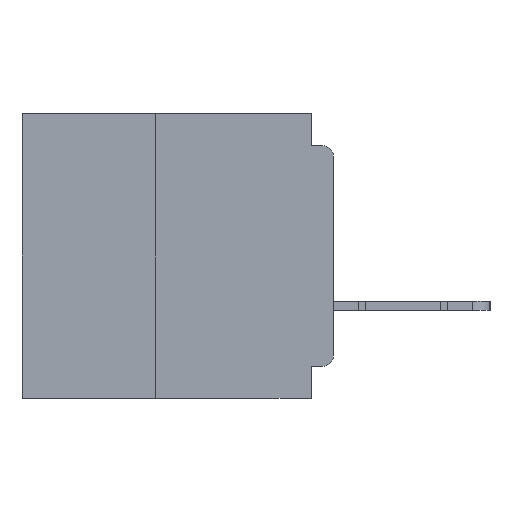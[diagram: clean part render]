
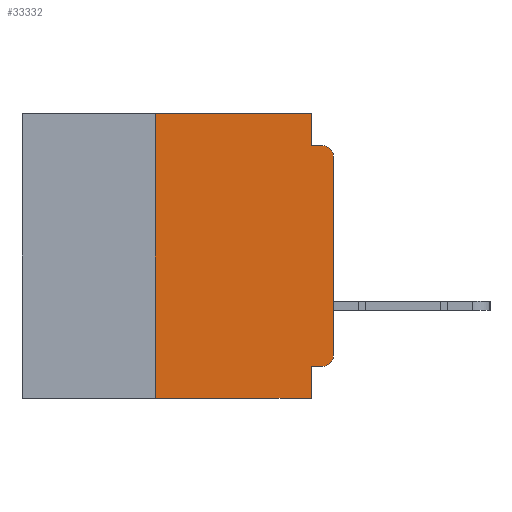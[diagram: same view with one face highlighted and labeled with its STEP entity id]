
A CAD part, left-side view. The second image highlights one B-rep face of the part: STEP entity #33332.
In plain terms, the highlighted planar face has unit normal (-1, 0, 0).
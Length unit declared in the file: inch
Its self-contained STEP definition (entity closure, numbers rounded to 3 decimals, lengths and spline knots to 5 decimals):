
#23 = VECTOR ( 'NONE', #9701, 39.37008 ) ;
#834 = EDGE_CURVE ( 'NONE', #57374, #1180, #47469, .T. ) ;
#1180 = VERTEX_POINT ( 'NONE', #57865 ) ;
#1313 = EDGE_CURVE ( 'NONE', #57374, #57992, #45757, .T. ) ;
#1717 = LINE ( 'NONE', #67734, #23 ) ;
#3343 = VECTOR ( 'NONE', #42000, 39.37008 ) ;
#3476 = DIRECTION ( 'NONE',  ( 0., 0., 1. ) ) ;
#3746 = DIRECTION ( 'NONE',  ( 0., 0., -1. ) ) ;
#3968 = DIRECTION ( 'NONE',  ( -1., 0., 0. ) ) ;
#3980 = CARTESIAN_POINT ( 'NONE',  ( 0., 0.015, -0.34 ) ) ;
#4348 = CARTESIAN_POINT ( 'NONE',  ( 0., 0.015, -0.045 ) ) ;
#5704 = CARTESIAN_POINT ( 'NONE',  ( 0., 0.031, -0.4 ) ) ;
#5742 = VERTEX_POINT ( 'NONE', #41278 ) ;
#6002 = ORIENTED_EDGE ( 'NONE', *, *, #11549, .T. ) ;
#6520 = EDGE_CURVE ( 'NONE', #5742, #25308, #28295, .T. ) ;
#7886 = VERTEX_POINT ( 'NONE', #61480 ) ;
#9701 = DIRECTION ( 'NONE',  ( 0., -1., 0. ) ) ;
#11549 = EDGE_CURVE ( 'NONE', #58336, #25308, #24708, .T. ) ;
#12817 = LINE ( 'NONE', #5704, #64125 ) ;
#13571 = EDGE_CURVE ( 'NONE', #1180, #58336, #45161, .T. ) ;
#14651 = VERTEX_POINT ( 'NONE', #18048 ) ;
#15087 = VECTOR ( 'NONE', #3476, 39.37008 ) ;
#15873 = VECTOR ( 'NONE', #26527, 39.37008 ) ;
#16516 = EDGE_CURVE ( 'NONE', #57992, #7886, #12817, .T. ) ;
#16991 = VECTOR ( 'NONE', #24159, 39.37008 ) ;
#17521 = CARTESIAN_POINT ( 'NONE',  ( 0., 0.031, 0. ) ) ;
#18048 = CARTESIAN_POINT ( 'NONE',  ( 0., 0.25, 0. ) ) ;
#21211 = CARTESIAN_POINT ( 'NONE',  ( 0., 0., -0.045 ) ) ;
#21913 = DIRECTION ( 'NONE',  ( 1., 0., 0. ) ) ;
#22072 = EDGE_CURVE ( 'NONE', #51188, #7886, #1717, .T. ) ;
#24159 = DIRECTION ( 'NONE',  ( 0., 0., 1. ) ) ;
#24708 = CIRCLE ( 'NONE', #51439, 0.015 ) ;
#25308 = VERTEX_POINT ( 'NONE', #4348 ) ;
#25977 = CARTESIAN_POINT ( 'NONE',  ( 0., 0.015, -0.355 ) ) ;
#26128 = CARTESIAN_POINT ( 'NONE',  ( 0., 0.031, -0.355 ) ) ;
#26527 = DIRECTION ( 'NONE',  ( 0., -1., 0. ) ) ;
#26719 = ORIENTED_EDGE ( 'NONE', *, *, #1313, .F. ) ;
#27508 = DIRECTION ( 'NONE',  ( 0., -1., 0. ) ) ;
#27667 = ORIENTED_EDGE ( 'NONE', *, *, #13571, .T. ) ;
#28295 = LINE ( 'NONE', #21211, #15873 ) ;
#30493 = AXIS2_PLACEMENT_3D ( 'NONE', #43035, #21913, #58931 ) ;
#31393 = CARTESIAN_POINT ( 'NONE',  ( 0., 0.015, -0.06 ) ) ;
#32190 = CARTESIAN_POINT ( 'NONE',  ( 0., 0.25, -0.4 ) ) ;
#33332 = ADVANCED_FACE ( 'NONE', ( #68121 ), #37674, .F. ) ;
#34059 = ORIENTED_EDGE ( 'NONE', *, *, #54883, .F. ) ;
#35324 = CARTESIAN_POINT ( 'NONE',  ( 0., 0.25, -0.4 ) ) ;
#36691 = DIRECTION ( 'NONE',  ( 0., 0., -1. ) ) ;
#37674 = PLANE ( 'NONE',  #30493 ) ;
#37801 = CARTESIAN_POINT ( 'NONE',  ( 0., 0.031, 0. ) ) ;
#38190 = ORIENTED_EDGE ( 'NONE', *, *, #16516, .F. ) ;
#38556 = ORIENTED_EDGE ( 'NONE', *, *, #6520, .F. ) ;
#39823 = ORIENTED_EDGE ( 'NONE', *, *, #22072, .T. ) ;
#39883 = CARTESIAN_POINT ( 'NONE',  ( 0., 0., -0.06 ) ) ;
#41278 = CARTESIAN_POINT ( 'NONE',  ( 0., 0.031, -0.045 ) ) ;
#42000 = DIRECTION ( 'NONE',  ( 0., 1., 0. ) ) ;
#42846 = DIRECTION ( 'NONE',  ( 0., 0., -1. ) ) ;
#43035 = CARTESIAN_POINT ( 'NONE',  ( 0., 0.437, 0. ) ) ;
#43056 = ORIENTED_EDGE ( 'NONE', *, *, #50293, .F. ) ;
#43297 = LINE ( 'NONE', #35324, #15087 ) ;
#45161 = LINE ( 'NONE', #50573, #16991 ) ;
#45404 = ORIENTED_EDGE ( 'NONE', *, *, #62286, .F. ) ;
#45757 = LINE ( 'NONE', #49192, #3343 ) ;
#47469 = CIRCLE ( 'NONE', #58877, 0.015 ) ;
#48051 = VECTOR ( 'NONE', #27508, 39.37008 ) ;
#48603 = CARTESIAN_POINT ( 'NONE',  ( 0., 0.437, 0. ) ) ;
#49192 = CARTESIAN_POINT ( 'NONE',  ( 0., 0., -0.355 ) ) ;
#50293 = EDGE_CURVE ( 'NONE', #51188, #14651, #43297, .T. ) ;
#50573 = CARTESIAN_POINT ( 'NONE',  ( 0., 0., 0. ) ) ;
#51188 = VERTEX_POINT ( 'NONE', #32190 ) ;
#51439 = AXIS2_PLACEMENT_3D ( 'NONE', #31393, #68248, #36691 ) ;
#52273 = EDGE_LOOP ( 'NONE', ( #27667, #6002, #38556, #45404, #34059, #43056, #39823, #38190, #26719, #58868 ) ) ;
#53125 = VECTOR ( 'NONE', #59045, 39.37008 ) ;
#54763 = LINE ( 'NONE', #37801, #53125 ) ;
#54883 = EDGE_CURVE ( 'NONE', #14651, #66091, #62031, .T. ) ;
#57374 = VERTEX_POINT ( 'NONE', #25977 ) ;
#57865 = CARTESIAN_POINT ( 'NONE',  ( 0., 0., -0.34 ) ) ;
#57992 = VERTEX_POINT ( 'NONE', #26128 ) ;
#58336 = VERTEX_POINT ( 'NONE', #39883 ) ;
#58868 = ORIENTED_EDGE ( 'NONE', *, *, #834, .T. ) ;
#58877 = AXIS2_PLACEMENT_3D ( 'NONE', #3980, #3968, #3746 ) ;
#58931 = DIRECTION ( 'NONE',  ( 0., 0., -1. ) ) ;
#59045 = DIRECTION ( 'NONE',  ( 0., 0., -1. ) ) ;
#61480 = CARTESIAN_POINT ( 'NONE',  ( 0., 0.031, -0.4 ) ) ;
#62031 = LINE ( 'NONE', #48603, #48051 ) ;
#62286 = EDGE_CURVE ( 'NONE', #66091, #5742, #54763, .T. ) ;
#64125 = VECTOR ( 'NONE', #42846, 39.37008 ) ;
#66091 = VERTEX_POINT ( 'NONE', #17521 ) ;
#67734 = CARTESIAN_POINT ( 'NONE',  ( 0., 0.437, -0.4 ) ) ;
#68121 = FACE_OUTER_BOUND ( 'NONE', #52273, .T. ) ;
#68248 = DIRECTION ( 'NONE',  ( -1., 0., 0. ) ) ;
